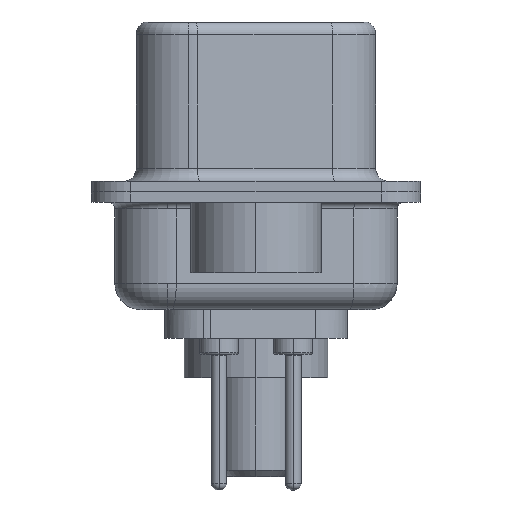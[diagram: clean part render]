
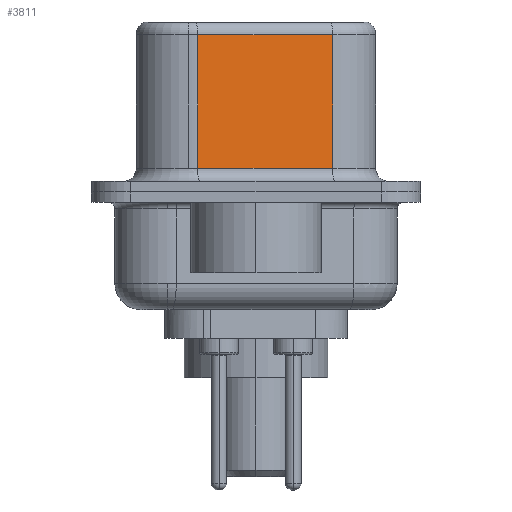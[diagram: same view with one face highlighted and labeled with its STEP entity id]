
A CAD part, left-side view. The second image highlights one B-rep face of the part: STEP entity #3811.
In plain terms, the highlighted planar face has unit normal (-0.985, -0.174, 0).
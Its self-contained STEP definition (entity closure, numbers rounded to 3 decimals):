
#409 = LINE ( 'NONE', #7913, #3905 ) ;
#555 = VECTOR ( 'NONE', #4469, 1000. ) ;
#1184 = DIRECTION ( 'NONE',  ( -0.174, 0.985, 0. ) ) ;
#2709 = ORIENTED_EDGE ( 'NONE', *, *, #19765, .T. ) ;
#3811 = ADVANCED_FACE ( 'NONE', ( #11001 ), #5649, .F. ) ;
#3905 = VECTOR ( 'NONE', #6364, 1000. ) ;
#4071 = VECTOR ( 'NONE', #10433, 1000. ) ;
#4469 = DIRECTION ( 'NONE',  ( 0., 0., -1. ) ) ;
#5402 = VERTEX_POINT ( 'NONE', #12498 ) ;
#5640 = CARTESIAN_POINT ( 'NONE',  ( 4.565, -2.927, 6.02 ) ) ;
#5649 = PLANE ( 'NONE',  #9047 ) ;
#5776 = CARTESIAN_POINT ( 'NONE',  ( 4.565, -2.927, 6.52 ) ) ;
#6364 = DIRECTION ( 'NONE',  ( 0.174, -0.985, 0. ) ) ;
#6722 = DIRECTION ( 'NONE',  ( 0.985, 0.174, 0. ) ) ;
#7913 = CARTESIAN_POINT ( 'NONE',  ( 4.565, -2.927, 0.9 ) ) ;
#8085 = LINE ( 'NONE', #19729, #4071 ) ;
#8435 = EDGE_CURVE ( 'NONE', #16225, #5402, #8085, .T. ) ;
#8965 = EDGE_CURVE ( 'NONE', #13186, #9076, #16774, .T. ) ;
#9047 = AXIS2_PLACEMENT_3D ( 'NONE', #5776, #6722, #12104 ) ;
#9076 = VERTEX_POINT ( 'NONE', #12302 ) ;
#10433 = DIRECTION ( 'NONE',  ( 0., 0., -1. ) ) ;
#11001 = FACE_OUTER_BOUND ( 'NONE', #11181, .T. ) ;
#11181 = EDGE_LOOP ( 'NONE', ( #14457, #19486, #17909, #2709 ) ) ;
#12104 = DIRECTION ( 'NONE',  ( -0.174, 0.985, 0. ) ) ;
#12302 = CARTESIAN_POINT ( 'NONE',  ( 4.565, -2.927, 0.9 ) ) ;
#12498 = CARTESIAN_POINT ( 'NONE',  ( 3.655, 2.233, 0.9 ) ) ;
#12867 = CARTESIAN_POINT ( 'NONE',  ( 3.655, 2.233, 6.02 ) ) ;
#13186 = VERTEX_POINT ( 'NONE', #14218 ) ;
#13675 = CARTESIAN_POINT ( 'NONE',  ( 4.565, -2.927, 6.52 ) ) ;
#14218 = CARTESIAN_POINT ( 'NONE',  ( 4.565, -2.927, 6.02 ) ) ;
#14457 = ORIENTED_EDGE ( 'NONE', *, *, #8965, .F. ) ;
#14567 = LINE ( 'NONE', #5640, #18178 ) ;
#15037 = EDGE_CURVE ( 'NONE', #13186, #16225, #14567, .T. ) ;
#16225 = VERTEX_POINT ( 'NONE', #12867 ) ;
#16774 = LINE ( 'NONE', #13675, #555 ) ;
#17909 = ORIENTED_EDGE ( 'NONE', *, *, #8435, .T. ) ;
#18178 = VECTOR ( 'NONE', #1184, 1000. ) ;
#19486 = ORIENTED_EDGE ( 'NONE', *, *, #15037, .T. ) ;
#19729 = CARTESIAN_POINT ( 'NONE',  ( 3.655, 2.233, 6.52 ) ) ;
#19765 = EDGE_CURVE ( 'NONE', #5402, #9076, #409, .T. ) ;
